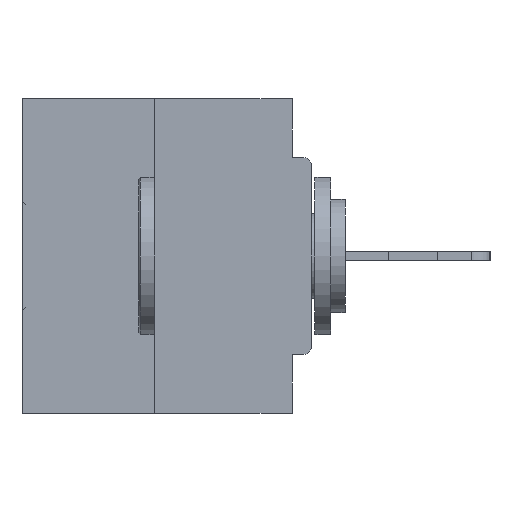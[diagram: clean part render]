
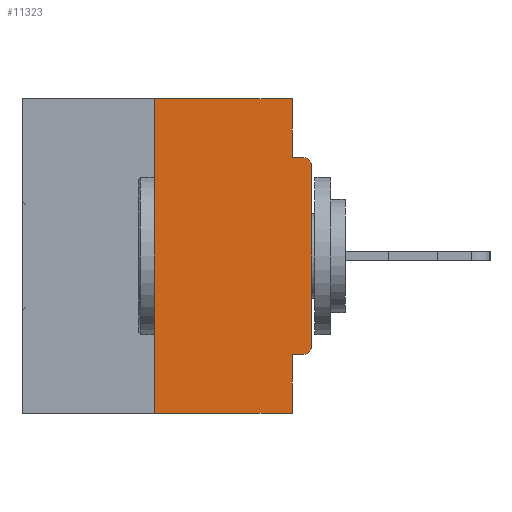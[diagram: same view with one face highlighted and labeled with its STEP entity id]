
A CAD part, left-side view. The second image highlights one B-rep face of the part: STEP entity #11323.
In plain terms, the highlighted planar face has unit normal (-1, 0, 0).
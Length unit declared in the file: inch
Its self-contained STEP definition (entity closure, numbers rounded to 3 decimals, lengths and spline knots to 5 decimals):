
#238 = LINE ( 'NONE', #6235, #24551 ) ;
#624 = DIRECTION ( 'NONE',  ( 0., 0., -1. ) ) ;
#1087 = ORIENTED_EDGE ( 'NONE', *, *, #19382, .F. ) ;
#1248 = VECTOR ( 'NONE', #19087, 39.37008 ) ;
#1568 = CARTESIAN_POINT ( 'NONE',  ( 0., 0.015, -0.0935 ) ) ;
#1592 = DIRECTION ( 'NONE',  ( 0., 0., 1. ) ) ;
#1688 = DIRECTION ( 'NONE',  ( 0., -1., 0. ) ) ;
#2094 = EDGE_CURVE ( 'NONE', #8297, #22648, #10049, .T. ) ;
#3502 = FACE_OUTER_BOUND ( 'NONE', #5675, .T. ) ;
#4171 = CIRCLE ( 'NONE', #25676, 0.015 ) ;
#5301 = CARTESIAN_POINT ( 'NONE',  ( 0., 0.015, -0.4065 ) ) ;
#5675 = EDGE_LOOP ( 'NONE', ( #10921, #36666, #20697, #1087, #30183, #8510, #28332, #7773, #13591, #33059 ) ) ;
#5733 = CARTESIAN_POINT ( 'NONE',  ( 0., 0.25, -0.5 ) ) ;
#6235 = CARTESIAN_POINT ( 'NONE',  ( 0., 0., -0.0935 ) ) ;
#7190 = CARTESIAN_POINT ( 'NONE',  ( 0., 0.031, -0.5 ) ) ;
#7264 = CARTESIAN_POINT ( 'NONE',  ( 0., 0., 0. ) ) ;
#7362 = VERTEX_POINT ( 'NONE', #30056 ) ;
#7773 = ORIENTED_EDGE ( 'NONE', *, *, #14631, .T. ) ;
#8297 = VERTEX_POINT ( 'NONE', #5301 ) ;
#8510 = ORIENTED_EDGE ( 'NONE', *, *, #34638, .T. ) ;
#9896 = VERTEX_POINT ( 'NONE', #20260 ) ;
#10049 = LINE ( 'NONE', #21960, #1248 ) ;
#10163 = VERTEX_POINT ( 'NONE', #24255 ) ;
#10484 = LINE ( 'NONE', #15840, #20231 ) ;
#10834 = CARTESIAN_POINT ( 'NONE',  ( 0., 0., -0.3915 ) ) ;
#10921 = ORIENTED_EDGE ( 'NONE', *, *, #26121, .F. ) ;
#10952 = LINE ( 'NONE', #33625, #15900 ) ;
#11323 = ADVANCED_FACE ( 'NONE', ( #3502 ), #20626, .F. ) ;
#11334 = EDGE_CURVE ( 'NONE', #10163, #20768, #238, .T. ) ;
#11819 = EDGE_CURVE ( 'NONE', #36301, #22124, #17003, .T. ) ;
#12556 = CARTESIAN_POINT ( 'NONE',  ( 0., 0.031, 0. ) ) ;
#13591 = ORIENTED_EDGE ( 'NONE', *, *, #11334, .F. ) ;
#13690 = CARTESIAN_POINT ( 'NONE',  ( 0., 0.015, -0.3915 ) ) ;
#14111 = VECTOR ( 'NONE', #16818, 39.37008 ) ;
#14256 = DIRECTION ( 'NONE',  ( 0., 0., -1. ) ) ;
#14631 = EDGE_CURVE ( 'NONE', #7362, #20768, #24337, .T. ) ;
#14787 = CARTESIAN_POINT ( 'NONE',  ( 0., 0.031, -0.4065 ) ) ;
#15616 = VECTOR ( 'NONE', #16446, 39.37008 ) ;
#15840 = CARTESIAN_POINT ( 'NONE',  ( 0., 0.25, 0. ) ) ;
#15877 = LINE ( 'NONE', #7264, #15616 ) ;
#15900 = VECTOR ( 'NONE', #1688, 39.37008 ) ;
#16446 = DIRECTION ( 'NONE',  ( 0., 0., 1. ) ) ;
#16818 = DIRECTION ( 'NONE',  ( 0., -1., 0. ) ) ;
#17003 = LINE ( 'NONE', #20283, #14111 ) ;
#18536 = VERTEX_POINT ( 'NONE', #10834 ) ;
#19087 = DIRECTION ( 'NONE',  ( 0., 1., 0. ) ) ;
#19382 = EDGE_CURVE ( 'NONE', #22648, #22124, #22166, .T. ) ;
#19454 = VECTOR ( 'NONE', #36562, 39.37008 ) ;
#19664 = DIRECTION ( 'NONE',  ( -1., 0., 0. ) ) ;
#20231 = VECTOR ( 'NONE', #1592, 39.37008 ) ;
#20260 = CARTESIAN_POINT ( 'NONE',  ( 0., 0.25, 0. ) ) ;
#20283 = CARTESIAN_POINT ( 'NONE',  ( 0., 0.46, -0.5 ) ) ;
#20626 = PLANE ( 'NONE',  #26994 ) ;
#20697 = ORIENTED_EDGE ( 'NONE', *, *, #11819, .T. ) ;
#20768 = VERTEX_POINT ( 'NONE', #1568 ) ;
#21190 = DIRECTION ( 'NONE',  ( 1., 0., 0. ) ) ;
#21573 = EDGE_CURVE ( 'NONE', #18536, #7362, #15877, .T. ) ;
#21960 = CARTESIAN_POINT ( 'NONE',  ( 0., 0., -0.4065 ) ) ;
#22124 = VERTEX_POINT ( 'NONE', #37163 ) ;
#22166 = LINE ( 'NONE', #7190, #19454 ) ;
#22648 = VERTEX_POINT ( 'NONE', #14787 ) ;
#24255 = CARTESIAN_POINT ( 'NONE',  ( 0., 0.031, -0.0935 ) ) ;
#24337 = CIRCLE ( 'NONE', #24930, 0.015 ) ;
#24551 = VECTOR ( 'NONE', #29672, 39.37008 ) ;
#24930 = AXIS2_PLACEMENT_3D ( 'NONE', #36633, #33383, #27989 ) ;
#25676 = AXIS2_PLACEMENT_3D ( 'NONE', #13690, #19664, #14256 ) ;
#26121 = EDGE_CURVE ( 'NONE', #9896, #29152, #10952, .T. ) ;
#26878 = EDGE_CURVE ( 'NONE', #36301, #9896, #10484, .T. ) ;
#26994 = AXIS2_PLACEMENT_3D ( 'NONE', #35827, #21190, #624 ) ;
#27047 = DIRECTION ( 'NONE',  ( 0., 0., -1. ) ) ;
#27989 = DIRECTION ( 'NONE',  ( 0., 0., -1. ) ) ;
#28332 = ORIENTED_EDGE ( 'NONE', *, *, #21573, .T. ) ;
#29152 = VERTEX_POINT ( 'NONE', #12556 ) ;
#29672 = DIRECTION ( 'NONE',  ( 0., -1., 0. ) ) ;
#30056 = CARTESIAN_POINT ( 'NONE',  ( 0., 0., -0.1085 ) ) ;
#30183 = ORIENTED_EDGE ( 'NONE', *, *, #2094, .F. ) ;
#31403 = EDGE_CURVE ( 'NONE', #29152, #10163, #35703, .T. ) ;
#31959 = VECTOR ( 'NONE', #27047, 39.37008 ) ;
#32801 = CARTESIAN_POINT ( 'NONE',  ( 0., 0.031, 0. ) ) ;
#33059 = ORIENTED_EDGE ( 'NONE', *, *, #31403, .F. ) ;
#33383 = DIRECTION ( 'NONE',  ( -1., 0., 0. ) ) ;
#33625 = CARTESIAN_POINT ( 'NONE',  ( 0., 0.46, 0. ) ) ;
#34638 = EDGE_CURVE ( 'NONE', #8297, #18536, #4171, .T. ) ;
#35703 = LINE ( 'NONE', #32801, #31959 ) ;
#35827 = CARTESIAN_POINT ( 'NONE',  ( 0., 0.46, 0. ) ) ;
#36301 = VERTEX_POINT ( 'NONE', #5733 ) ;
#36562 = DIRECTION ( 'NONE',  ( 0., 0., -1. ) ) ;
#36633 = CARTESIAN_POINT ( 'NONE',  ( 0., 0.015, -0.1085 ) ) ;
#36666 = ORIENTED_EDGE ( 'NONE', *, *, #26878, .F. ) ;
#37163 = CARTESIAN_POINT ( 'NONE',  ( 0., 0.031, -0.5 ) ) ;
